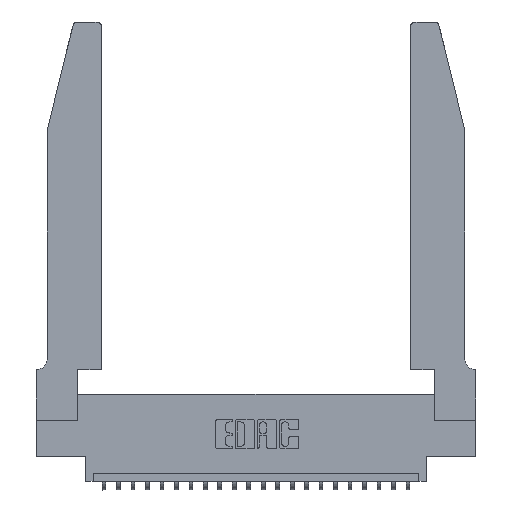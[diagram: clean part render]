
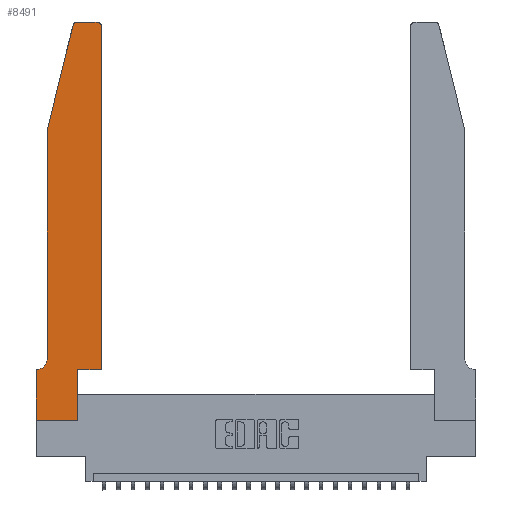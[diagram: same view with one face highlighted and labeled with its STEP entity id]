
A CAD part, top view. The second image highlights one B-rep face of the part: STEP entity #8491.
In plain terms, the highlighted planar face has unit normal (0, 0, 1).
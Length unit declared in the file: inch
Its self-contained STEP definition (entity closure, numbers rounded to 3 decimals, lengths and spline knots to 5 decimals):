
#131 = CARTESIAN_POINT ( 'NONE',  ( 0.2605, 2.75, 0.37 ) ) ;
#267 = EDGE_CURVE ( 'NONE', #12279, #3583, #8507, .T. ) ;
#409 = ORIENTED_EDGE ( 'NONE', *, *, #9501, .T. ) ;
#749 = ORIENTED_EDGE ( 'NONE', *, *, #7346, .T. ) ;
#1270 = VECTOR ( 'NONE', #17984, 39.37008 ) ;
#1289 = ORIENTED_EDGE ( 'NONE', *, *, #3946, .T. ) ;
#1755 = CARTESIAN_POINT ( 'NONE',  ( 0.4505, 2.72, 0.37 ) ) ;
#1794 = ORIENTED_EDGE ( 'NONE', *, *, #14358, .T. ) ;
#2065 = VECTOR ( 'NONE', #7777, 39.37008 ) ;
#2216 = VERTEX_POINT ( 'NONE', #24110 ) ;
#2250 = CARTESIAN_POINT ( 'NONE',  ( 0.0055, 0.35, 0.37 ) ) ;
#2511 = DIRECTION ( 'NONE',  ( 0., -1., 0. ) ) ;
#2525 = CARTESIAN_POINT ( 'NONE',  ( 0.4205, 2.72, 0.37 ) ) ;
#2608 = DIRECTION ( 'NONE',  ( 0., 0., 1. ) ) ;
#2957 = CARTESIAN_POINT ( 'NONE',  ( 0.284, 2.72, 0.37 ) ) ;
#3186 = VERTEX_POINT ( 'NONE', #14760 ) ;
#3205 = VECTOR ( 'NONE', #5100, 39.37008 ) ;
#3219 = DIRECTION ( 'NONE',  ( -1., 0., 0. ) ) ;
#3583 = VERTEX_POINT ( 'NONE', #5715 ) ;
#3937 = AXIS2_PLACEMENT_3D ( 'NONE', #20473, #16563, #22355 ) ;
#3946 = EDGE_CURVE ( 'NONE', #16076, #3186, #6597, .T. ) ;
#4357 = ORIENTED_EDGE ( 'NONE', *, *, #12296, .T. ) ;
#4497 = VERTEX_POINT ( 'NONE', #2250 ) ;
#4891 = DIRECTION ( 'NONE',  ( 1., 0., 0. ) ) ;
#5100 = DIRECTION ( 'NONE',  ( 0., -1., 0. ) ) ;
#5246 = LINE ( 'NONE', #10818, #11679 ) ;
#5572 = VERTEX_POINT ( 'NONE', #9524 ) ;
#5674 = ORIENTED_EDGE ( 'NONE', *, *, #21494, .T. ) ;
#5715 = CARTESIAN_POINT ( 'NONE',  ( 0.284, 2.75, 0.37 ) ) ;
#5814 = LINE ( 'NONE', #12541, #3205 ) ;
#6252 = AXIS2_PLACEMENT_3D ( 'NONE', #2525, #2608, #15711 ) ;
#6597 = LINE ( 'NONE', #15343, #24184 ) ;
#6840 = CARTESIAN_POINT ( 'NONE',  ( 0., 0., 0.37 ) ) ;
#7300 = CARTESIAN_POINT ( 'NONE',  ( 0.0755, 2., 0.37 ) ) ;
#7346 = EDGE_CURVE ( 'NONE', #11512, #12279, #13230, .T. ) ;
#7417 = ORIENTED_EDGE ( 'NONE', *, *, #267, .T. ) ;
#7777 = DIRECTION ( 'NONE',  ( -1., 0., 0. ) ) ;
#7898 = CARTESIAN_POINT ( 'NONE',  ( 0., 0.35, 0.37 ) ) ;
#8179 = CARTESIAN_POINT ( 'NONE',  ( 0.4505, 0.35, 0.37 ) ) ;
#8491 = ADVANCED_FACE ( 'NONE', ( #19667 ), #16329, .T. ) ;
#8507 = LINE ( 'NONE', #131, #2065 ) ;
#8710 = VERTEX_POINT ( 'NONE', #13225 ) ;
#8796 = CARTESIAN_POINT ( 'NONE',  ( 0.0755, 0.35, 0.37 ) ) ;
#9475 = EDGE_CURVE ( 'NONE', #8710, #11512, #5246, .T. ) ;
#9501 = EDGE_CURVE ( 'NONE', #5572, #20992, #5814, .T. ) ;
#9524 = CARTESIAN_POINT ( 'NONE',  ( 0.0755, 2., 0.37 ) ) ;
#10067 = CARTESIAN_POINT ( 'NONE',  ( 0.4205, 2.75, 0.37 ) ) ;
#10069 = DIRECTION ( 'NONE',  ( 1., 0., 0. ) ) ;
#10141 = CIRCLE ( 'NONE', #3937, 0.07 ) ;
#10818 = CARTESIAN_POINT ( 'NONE',  ( 0.4505, 0.35, 0.37 ) ) ;
#11196 = CARTESIAN_POINT ( 'NONE',  ( 0., 0.35, 0.37 ) ) ;
#11286 = DIRECTION ( 'NONE',  ( -0.239, -0.971, 0. ) ) ;
#11288 = VECTOR ( 'NONE', #3219, 39.37008 ) ;
#11512 = VERTEX_POINT ( 'NONE', #1755 ) ;
#11679 = VECTOR ( 'NONE', #24040, 39.37008 ) ;
#11926 = VERTEX_POINT ( 'NONE', #14596 ) ;
#12000 = ORIENTED_EDGE ( 'NONE', *, *, #17836, .T. ) ;
#12279 = VERTEX_POINT ( 'NONE', #10067 ) ;
#12296 = EDGE_CURVE ( 'NONE', #11926, #14745, #19996, .T. ) ;
#12541 = CARTESIAN_POINT ( 'NONE',  ( 0.0755, 2., 0.37 ) ) ;
#12992 = DIRECTION ( 'NONE',  ( 0., 0., 1. ) ) ;
#13111 = LINE ( 'NONE', #8179, #22804 ) ;
#13225 = CARTESIAN_POINT ( 'NONE',  ( 0.4505, 0.35, 0.37 ) ) ;
#13230 = CIRCLE ( 'NONE', #6252, 0.03 ) ;
#14257 = EDGE_CURVE ( 'NONE', #14745, #8710, #13111, .T. ) ;
#14358 = EDGE_CURVE ( 'NONE', #3583, #2216, #15148, .T. ) ;
#14378 = ORIENTED_EDGE ( 'NONE', *, *, #9475, .T. ) ;
#14596 = CARTESIAN_POINT ( 'NONE',  ( 0.2865, 0., 0.37 ) ) ;
#14745 = VERTEX_POINT ( 'NONE', #16863 ) ;
#14760 = CARTESIAN_POINT ( 'NONE',  ( 0., 0., 0.37 ) ) ;
#14934 = AXIS2_PLACEMENT_3D ( 'NONE', #2957, #23588, #4891 ) ;
#15148 = CIRCLE ( 'NONE', #14934, 0.03 ) ;
#15343 = CARTESIAN_POINT ( 'NONE',  ( 0., 0., 0.37 ) ) ;
#15711 = DIRECTION ( 'NONE',  ( 1., 0., 0. ) ) ;
#15869 = LINE ( 'NONE', #6840, #21172 ) ;
#16076 = VERTEX_POINT ( 'NONE', #7898 ) ;
#16329 = PLANE ( 'NONE',  #23714 ) ;
#16431 = EDGE_CURVE ( 'NONE', #4497, #16076, #18920, .T. ) ;
#16563 = DIRECTION ( 'NONE',  ( 0., 0., -1. ) ) ;
#16863 = CARTESIAN_POINT ( 'NONE',  ( 0.2865, 0.35, 0.37 ) ) ;
#16869 = LINE ( 'NONE', #7300, #17183 ) ;
#17183 = VECTOR ( 'NONE', #11286, 39.37008 ) ;
#17836 = EDGE_CURVE ( 'NONE', #3186, #11926, #15869, .T. ) ;
#17984 = DIRECTION ( 'NONE',  ( 0., 1., 0. ) ) ;
#18920 = LINE ( 'NONE', #8796, #11288 ) ;
#19667 = FACE_OUTER_BOUND ( 'NONE', #20423, .T. ) ;
#19685 = CARTESIAN_POINT ( 'NONE',  ( 0.2865, 0.35, 0.37 ) ) ;
#19888 = DIRECTION ( 'NONE',  ( 1., 0., 0. ) ) ;
#19996 = LINE ( 'NONE', #19685, #1270 ) ;
#20423 = EDGE_LOOP ( 'NONE', ( #7417, #1794, #5674, #409, #22596, #20745, #1289, #12000, #4357, #24159, #14378, #749 ) ) ;
#20473 = CARTESIAN_POINT ( 'NONE',  ( 0.0055, 0.42, 0.37 ) ) ;
#20745 = ORIENTED_EDGE ( 'NONE', *, *, #16431, .T. ) ;
#20992 = VERTEX_POINT ( 'NONE', #22395 ) ;
#21172 = VECTOR ( 'NONE', #19888, 39.37008 ) ;
#21494 = EDGE_CURVE ( 'NONE', #2216, #5572, #16869, .T. ) ;
#22355 = DIRECTION ( 'NONE',  ( -1., 0., 0. ) ) ;
#22357 = DIRECTION ( 'NONE',  ( 1., 0., 0. ) ) ;
#22395 = CARTESIAN_POINT ( 'NONE',  ( 0.0755, 0.42, 0.37 ) ) ;
#22596 = ORIENTED_EDGE ( 'NONE', *, *, #24031, .T. ) ;
#22804 = VECTOR ( 'NONE', #10069, 39.37008 ) ;
#23588 = DIRECTION ( 'NONE',  ( 0., 0., 1. ) ) ;
#23714 = AXIS2_PLACEMENT_3D ( 'NONE', #11196, #12992, #22357 ) ;
#24031 = EDGE_CURVE ( 'NONE', #20992, #4497, #10141, .T. ) ;
#24040 = DIRECTION ( 'NONE',  ( 0., 1., 0. ) ) ;
#24110 = CARTESIAN_POINT ( 'NONE',  ( 0.25487, 2.72718, 0.37 ) ) ;
#24159 = ORIENTED_EDGE ( 'NONE', *, *, #14257, .T. ) ;
#24184 = VECTOR ( 'NONE', #2511, 39.37008 ) ;
